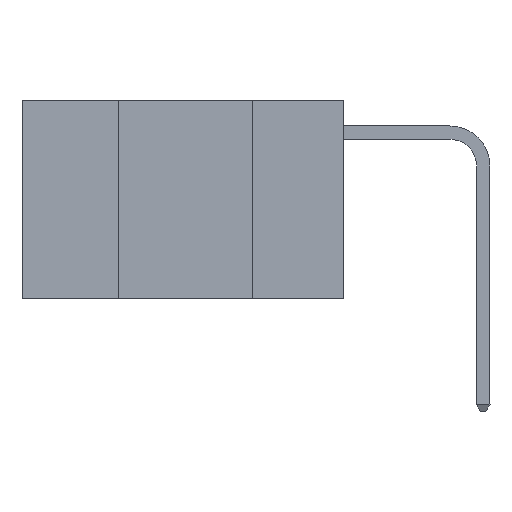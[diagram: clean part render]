
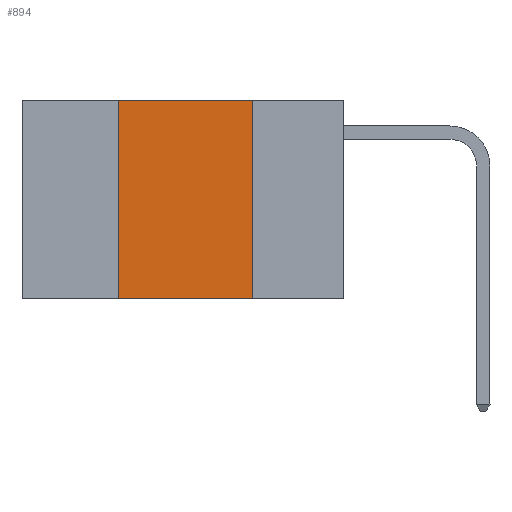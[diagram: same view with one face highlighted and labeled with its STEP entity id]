
A CAD part, left-side view. The second image highlights one B-rep face of the part: STEP entity #894.
In plain terms, the highlighted planar face has unit normal (-1, 0, 0).
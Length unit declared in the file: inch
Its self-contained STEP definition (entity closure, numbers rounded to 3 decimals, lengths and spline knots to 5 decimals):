
#771 = CARTESIAN_POINT ( 'NONE',  ( 0., 0.42, 0. ) ) ;
#894 = ADVANCED_FACE ( 'NONE', ( #23340 ), #18875, .F. ) ;
#1060 = CARTESIAN_POINT ( 'NONE',  ( 0., 0.6, 0. ) ) ;
#2201 = CARTESIAN_POINT ( 'NONE',  ( 0., 0.6, 0. ) ) ;
#3271 = ORIENTED_EDGE ( 'NONE', *, *, #8200, .F. ) ;
#3520 = ORIENTED_EDGE ( 'NONE', *, *, #7677, .F. ) ;
#4468 = CARTESIAN_POINT ( 'NONE',  ( 0., 0.42, 0. ) ) ;
#4600 = LINE ( 'NONE', #12522, #23667 ) ;
#5054 = EDGE_CURVE ( 'NONE', #7940, #17525, #10786, .T. ) ;
#5341 = ORIENTED_EDGE ( 'NONE', *, *, #5054, .F. ) ;
#5750 = CARTESIAN_POINT ( 'NONE',  ( 0., 0.42, -0.37 ) ) ;
#7677 = EDGE_CURVE ( 'NONE', #12536, #9094, #4600, .T. ) ;
#7940 = VERTEX_POINT ( 'NONE', #5750 ) ;
#8200 = EDGE_CURVE ( 'NONE', #17525, #12536, #10027, .T. ) ;
#9094 = VERTEX_POINT ( 'NONE', #22923 ) ;
#9125 = VECTOR ( 'NONE', #10146, 39.37008 ) ;
#9150 = DIRECTION ( 'NONE',  ( 1., 0., 0. ) ) ;
#9739 = DIRECTION ( 'NONE',  ( 0., -1., 0. ) ) ;
#10027 = LINE ( 'NONE', #2201, #9125 ) ;
#10146 = DIRECTION ( 'NONE',  ( 0., -1., 0. ) ) ;
#10239 = VECTOR ( 'NONE', #24608, 39.37008 ) ;
#10573 = DIRECTION ( 'NONE',  ( 0., 0., -1. ) ) ;
#10786 = LINE ( 'NONE', #771, #10239 ) ;
#11416 = EDGE_CURVE ( 'NONE', #7940, #9094, #15570, .T. ) ;
#12522 = CARTESIAN_POINT ( 'NONE',  ( 0., 0.17, 0. ) ) ;
#12536 = VERTEX_POINT ( 'NONE', #15523 ) ;
#15523 = CARTESIAN_POINT ( 'NONE',  ( 0., 0.17, 0. ) ) ;
#15570 = LINE ( 'NONE', #19744, #16214 ) ;
#16214 = VECTOR ( 'NONE', #9739, 39.37008 ) ;
#17525 = VERTEX_POINT ( 'NONE', #4468 ) ;
#18875 = PLANE ( 'NONE',  #19922 ) ;
#19744 = CARTESIAN_POINT ( 'NONE',  ( 0., 0.6, -0.37 ) ) ;
#19922 = AXIS2_PLACEMENT_3D ( 'NONE', #1060, #9150, #22811 ) ;
#22811 = DIRECTION ( 'NONE',  ( 0., 0., -1. ) ) ;
#22923 = CARTESIAN_POINT ( 'NONE',  ( 0., 0.17, -0.37 ) ) ;
#22944 = EDGE_LOOP ( 'NONE', ( #3520, #3271, #5341, #23086 ) ) ;
#23086 = ORIENTED_EDGE ( 'NONE', *, *, #11416, .T. ) ;
#23340 = FACE_OUTER_BOUND ( 'NONE', #22944, .T. ) ;
#23667 = VECTOR ( 'NONE', #10573, 39.37008 ) ;
#24608 = DIRECTION ( 'NONE',  ( 0., 0., 1. ) ) ;
